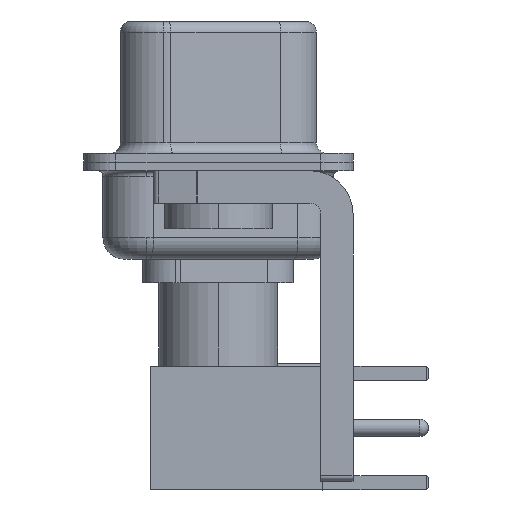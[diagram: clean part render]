
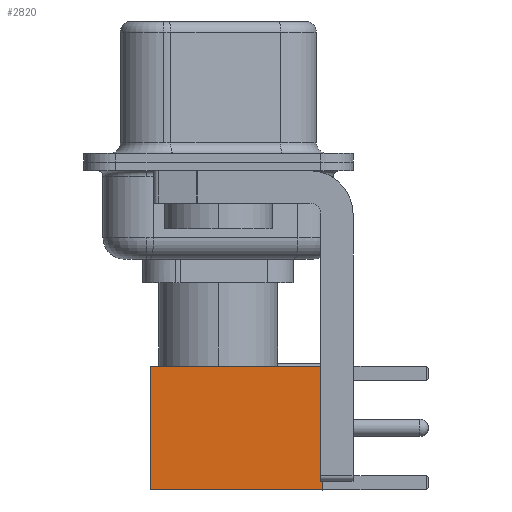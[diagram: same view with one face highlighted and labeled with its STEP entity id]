
A CAD part, left-side view. The second image highlights one B-rep face of the part: STEP entity #2820.
In plain terms, the highlighted face is planar.
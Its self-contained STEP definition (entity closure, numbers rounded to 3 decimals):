
#2820 = ADVANCED_FACE ( 'NONE', ( #16034 ), #15888, .T. ) ;
#3329 = CARTESIAN_POINT ( 'NONE',  ( 0., 2.875, 0. ) ) ;
#3580 = CARTESIAN_POINT ( 'NONE',  ( -2.875, 2.875, 0. ) ) ;
#3679 = EDGE_CURVE ( 'NONE', #12800, #16892, #7093, .T. ) ;
#4411 = EDGE_CURVE ( 'NONE', #16892, #15130, #9369, .T. ) ;
#4831 = DIRECTION ( 'NONE',  ( 0., 1., 0. ) ) ;
#4944 = DIRECTION ( 'NONE',  ( 0., 0., -1. ) ) ;
#5540 = VECTOR ( 'NONE', #4944, 1000. ) ;
#5550 = LINE ( 'NONE', #28527, #17961 ) ;
#6776 = EDGE_LOOP ( 'NONE', ( #21500, #28435, #22291, #22303 ) ) ;
#7093 = LINE ( 'NONE', #17594, #20104 ) ;
#9369 = LINE ( 'NONE', #14213, #5540 ) ;
#9726 = AXIS2_PLACEMENT_3D ( 'NONE', #24864, #4831, #19862 ) ;
#9963 = DIRECTION ( 'NONE',  ( -1., 0., 0. ) ) ;
#10091 = CARTESIAN_POINT ( 'NONE',  ( 2.875, 2.875, 0. ) ) ;
#12458 = DIRECTION ( 'NONE',  ( 0., 0., -1. ) ) ;
#12800 = VERTEX_POINT ( 'NONE', #16191 ) ;
#14213 = CARTESIAN_POINT ( 'NONE',  ( -2.875, 2.875, 0. ) ) ;
#14719 = VECTOR ( 'NONE', #9963, 1000. ) ;
#15130 = VERTEX_POINT ( 'NONE', #3580 ) ;
#15888 = PLANE ( 'NONE',  #9726 ) ;
#16034 = FACE_OUTER_BOUND ( 'NONE', #6776, .T. ) ;
#16191 = CARTESIAN_POINT ( 'NONE',  ( 2.875, 2.875, 8. ) ) ;
#16892 = VERTEX_POINT ( 'NONE', #24632 ) ;
#17594 = CARTESIAN_POINT ( 'NONE',  ( 0., 2.875, 8. ) ) ;
#17961 = VECTOR ( 'NONE', #12458, 1000. ) ;
#19049 = VERTEX_POINT ( 'NONE', #10091 ) ;
#19862 = DIRECTION ( 'NONE',  ( 0., 0., 1. ) ) ;
#20104 = VECTOR ( 'NONE', #24349, 1000. ) ;
#21500 = ORIENTED_EDGE ( 'NONE', *, *, #22795, .T. ) ;
#22291 = ORIENTED_EDGE ( 'NONE', *, *, #4411, .F. ) ;
#22303 = ORIENTED_EDGE ( 'NONE', *, *, #3679, .F. ) ;
#22795 = EDGE_CURVE ( 'NONE', #12800, #19049, #5550, .T. ) ;
#23789 = LINE ( 'NONE', #3329, #14719 ) ;
#24349 = DIRECTION ( 'NONE',  ( -1., 0., 0. ) ) ;
#24632 = CARTESIAN_POINT ( 'NONE',  ( -2.875, 2.875, 8. ) ) ;
#24864 = CARTESIAN_POINT ( 'NONE',  ( 2.875, 2.875, 0. ) ) ;
#25839 = EDGE_CURVE ( 'NONE', #19049, #15130, #23789, .T. ) ;
#28435 = ORIENTED_EDGE ( 'NONE', *, *, #25839, .T. ) ;
#28527 = CARTESIAN_POINT ( 'NONE',  ( 2.875, 2.875, 0. ) ) ;
